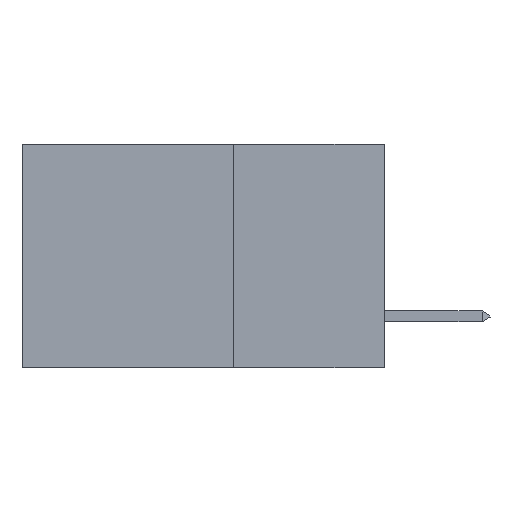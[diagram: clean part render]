
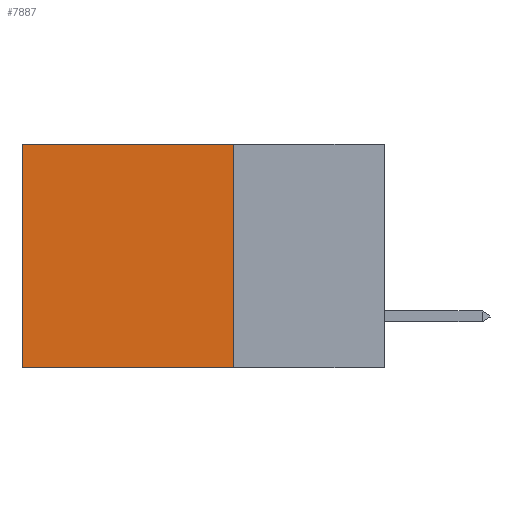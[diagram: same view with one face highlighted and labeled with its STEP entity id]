
A CAD part, left-side view. The second image highlights one B-rep face of the part: STEP entity #7887.
In plain terms, the highlighted planar face has unit normal (-1, 0, 0).
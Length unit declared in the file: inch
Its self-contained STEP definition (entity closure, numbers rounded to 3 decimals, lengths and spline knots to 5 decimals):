
#122 = VERTEX_POINT ( 'NONE', #6270 ) ;
#210 = VECTOR ( 'NONE', #7932, 39.37008 ) ;
#667 = ORIENTED_EDGE ( 'NONE', *, *, #6144, .F. ) ;
#1916 = EDGE_CURVE ( 'NONE', #8664, #3562, #10359, .T. ) ;
#2416 = EDGE_CURVE ( 'NONE', #122, #8664, #14705, .T. ) ;
#3007 = DIRECTION ( 'NONE',  ( 0., 0., -1. ) ) ;
#3482 = DIRECTION ( 'NONE',  ( 0., 1., 0. ) ) ;
#3562 = VERTEX_POINT ( 'NONE', #12579 ) ;
#4278 = EDGE_LOOP ( 'NONE', ( #11369, #667, #13192, #9077 ) ) ;
#5154 = LINE ( 'NONE', #12073, #14070 ) ;
#5249 = VECTOR ( 'NONE', #3482, 39.37008 ) ;
#5516 = FACE_OUTER_BOUND ( 'NONE', #4278, .T. ) ;
#6144 = EDGE_CURVE ( 'NONE', #7295, #3562, #5154, .T. ) ;
#6270 = CARTESIAN_POINT ( 'NONE',  ( 0.2875, 0.25, 0. ) ) ;
#7074 = DIRECTION ( 'NONE',  ( 0., 0., -1. ) ) ;
#7091 = EDGE_CURVE ( 'NONE', #122, #7295, #10200, .T. ) ;
#7295 = VERTEX_POINT ( 'NONE', #7334 ) ;
#7334 = CARTESIAN_POINT ( 'NONE',  ( 0.2875, 0.25, -0.37 ) ) ;
#7671 = PLANE ( 'NONE',  #8563 ) ;
#7887 = ADVANCED_FACE ( 'NONE', ( #5516 ), #7671, .F. ) ;
#7932 = DIRECTION ( 'NONE',  ( 0., 0., -1. ) ) ;
#8239 = CARTESIAN_POINT ( 'NONE',  ( 0.2875, 0.6, 0. ) ) ;
#8563 = AXIS2_PLACEMENT_3D ( 'NONE', #13496, #9960, #3007 ) ;
#8664 = VERTEX_POINT ( 'NONE', #14316 ) ;
#9077 = ORIENTED_EDGE ( 'NONE', *, *, #2416, .T. ) ;
#9960 = DIRECTION ( 'NONE',  ( 1., 0., 0. ) ) ;
#10200 = LINE ( 'NONE', #11154, #210 ) ;
#10359 = LINE ( 'NONE', #8239, #14014 ) ;
#10452 = CARTESIAN_POINT ( 'NONE',  ( 0.2875, 0.25, 0. ) ) ;
#11154 = CARTESIAN_POINT ( 'NONE',  ( 0.2875, 0.25, 0. ) ) ;
#11369 = ORIENTED_EDGE ( 'NONE', *, *, #1916, .T. ) ;
#12073 = CARTESIAN_POINT ( 'NONE',  ( 0.2875, 0.25, -0.37 ) ) ;
#12173 = DIRECTION ( 'NONE',  ( 0., 1., 0. ) ) ;
#12579 = CARTESIAN_POINT ( 'NONE',  ( 0.2875, 0.6, -0.37 ) ) ;
#13192 = ORIENTED_EDGE ( 'NONE', *, *, #7091, .F. ) ;
#13496 = CARTESIAN_POINT ( 'NONE',  ( 0.2875, 0.25, 0. ) ) ;
#14014 = VECTOR ( 'NONE', #7074, 39.37008 ) ;
#14070 = VECTOR ( 'NONE', #12173, 39.37008 ) ;
#14316 = CARTESIAN_POINT ( 'NONE',  ( 0.2875, 0.6, 0. ) ) ;
#14705 = LINE ( 'NONE', #10452, #5249 ) ;
